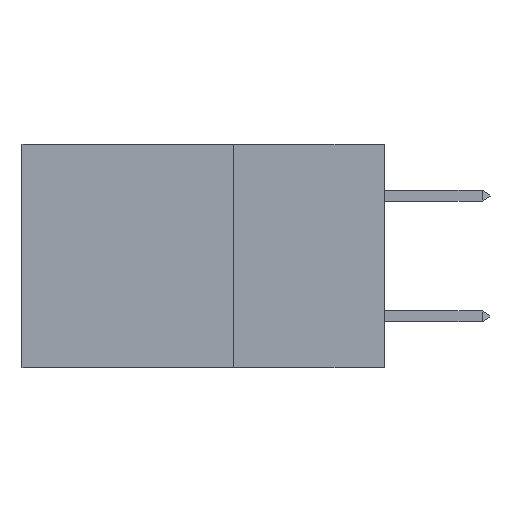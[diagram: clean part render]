
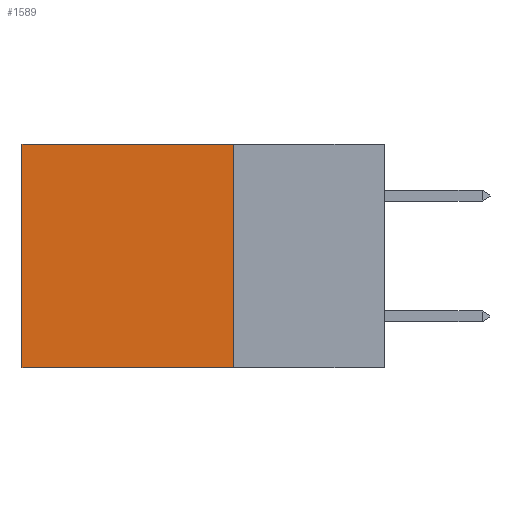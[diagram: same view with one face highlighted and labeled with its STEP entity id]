
A CAD part, left-side view. The second image highlights one B-rep face of the part: STEP entity #1589.
In plain terms, the highlighted planar face has unit normal (-1, 0, 0).
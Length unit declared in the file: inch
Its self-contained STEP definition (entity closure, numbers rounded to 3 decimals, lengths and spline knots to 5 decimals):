
#194 = DIRECTION ( 'NONE',  ( 0., 0., -1. ) ) ;
#318 = PLANE ( 'NONE',  #3981 ) ;
#984 = VECTOR ( 'NONE', #8077, 39.37008 ) ;
#1077 = DIRECTION ( 'NONE',  ( 0., 0., -1. ) ) ;
#1090 = CARTESIAN_POINT ( 'NONE',  ( 0.2875, 0.6, 0. ) ) ;
#1589 = ADVANCED_FACE ( 'NONE', ( #6091 ), #318, .F. ) ;
#1803 = EDGE_CURVE ( 'NONE', #3963, #2150, #5560, .T. ) ;
#1932 = DIRECTION ( 'NONE',  ( 0., 1., 0. ) ) ;
#2069 = ORIENTED_EDGE ( 'NONE', *, *, #5441, .F. ) ;
#2150 = VERTEX_POINT ( 'NONE', #8072 ) ;
#2426 = LINE ( 'NONE', #1090, #3431 ) ;
#2510 = CARTESIAN_POINT ( 'NONE',  ( 0.2875, 0.25, 0. ) ) ;
#2568 = DIRECTION ( 'NONE',  ( 0., 0., -1. ) ) ;
#3431 = VECTOR ( 'NONE', #2568, 39.37008 ) ;
#3730 = CARTESIAN_POINT ( 'NONE',  ( 0.2875, 0.25, -0.37 ) ) ;
#3776 = VERTEX_POINT ( 'NONE', #4679 ) ;
#3963 = VERTEX_POINT ( 'NONE', #6498 ) ;
#3981 = AXIS2_PLACEMENT_3D ( 'NONE', #2510, #6138, #1077 ) ;
#4290 = EDGE_LOOP ( 'NONE', ( #8053, #5034, #2069, #9390 ) ) ;
#4679 = CARTESIAN_POINT ( 'NONE',  ( 0.2875, 0.25, -0.37 ) ) ;
#5034 = ORIENTED_EDGE ( 'NONE', *, *, #6889, .F. ) ;
#5441 = EDGE_CURVE ( 'NONE', #3963, #3776, #8891, .T. ) ;
#5560 = LINE ( 'NONE', #8484, #8419 ) ;
#6091 = FACE_OUTER_BOUND ( 'NONE', #4290, .T. ) ;
#6138 = DIRECTION ( 'NONE',  ( 1., 0., 0. ) ) ;
#6300 = VECTOR ( 'NONE', #194, 39.37008 ) ;
#6498 = CARTESIAN_POINT ( 'NONE',  ( 0.2875, 0.25, 0. ) ) ;
#6548 = LINE ( 'NONE', #3730, #984 ) ;
#6889 = EDGE_CURVE ( 'NONE', #3776, #7199, #6548, .T. ) ;
#7199 = VERTEX_POINT ( 'NONE', #9426 ) ;
#7427 = EDGE_CURVE ( 'NONE', #2150, #7199, #2426, .T. ) ;
#8053 = ORIENTED_EDGE ( 'NONE', *, *, #7427, .T. ) ;
#8072 = CARTESIAN_POINT ( 'NONE',  ( 0.2875, 0.6, 0. ) ) ;
#8077 = DIRECTION ( 'NONE',  ( 0., 1., 0. ) ) ;
#8419 = VECTOR ( 'NONE', #1932, 39.37008 ) ;
#8484 = CARTESIAN_POINT ( 'NONE',  ( 0.2875, 0.25, 0. ) ) ;
#8891 = LINE ( 'NONE', #8990, #6300 ) ;
#8990 = CARTESIAN_POINT ( 'NONE',  ( 0.2875, 0.25, 0. ) ) ;
#9390 = ORIENTED_EDGE ( 'NONE', *, *, #1803, .T. ) ;
#9426 = CARTESIAN_POINT ( 'NONE',  ( 0.2875, 0.6, -0.37 ) ) ;
